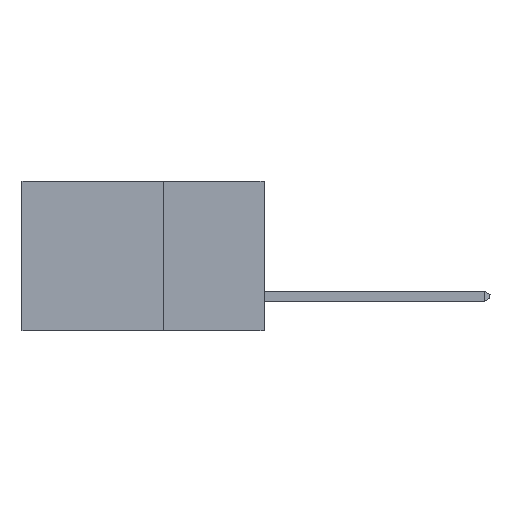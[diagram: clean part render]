
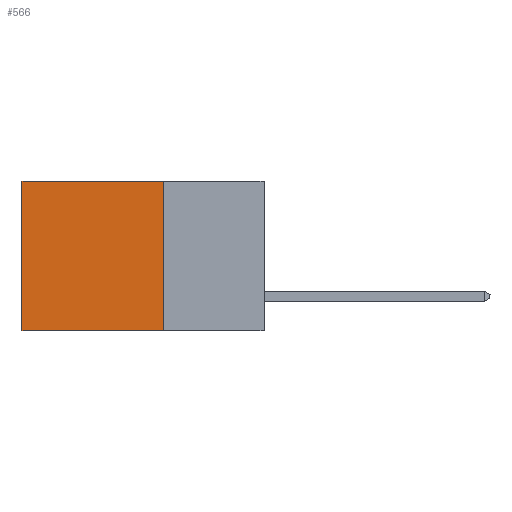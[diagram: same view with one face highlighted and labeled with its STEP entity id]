
A CAD part, left-side view. The second image highlights one B-rep face of the part: STEP entity #566.
In plain terms, the highlighted planar face has unit normal (-1, 0, 0).
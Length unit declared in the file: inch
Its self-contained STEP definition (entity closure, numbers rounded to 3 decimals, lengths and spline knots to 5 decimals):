
#61 = CARTESIAN_POINT ( 'NONE',  ( 0.298, 0.25, -0.37 ) ) ;
#566 = ADVANCED_FACE ( 'NONE', ( #7269 ), #3230, .F. ) ;
#623 = CARTESIAN_POINT ( 'NONE',  ( 0.298, 0.6, 0. ) ) ;
#704 = CARTESIAN_POINT ( 'NONE',  ( 0.298, 0.25, 0. ) ) ;
#1012 = DIRECTION ( 'NONE',  ( 0., 0., -1. ) ) ;
#1106 = LINE ( 'NONE', #704, #5927 ) ;
#1381 = ORIENTED_EDGE ( 'NONE', *, *, #5253, .F. ) ;
#2060 = EDGE_CURVE ( 'NONE', #2412, #5916, #2661, .T. ) ;
#2273 = DIRECTION ( 'NONE',  ( 0., 1., 0. ) ) ;
#2412 = VERTEX_POINT ( 'NONE', #61 ) ;
#2661 = LINE ( 'NONE', #9567, #9022 ) ;
#2744 = VECTOR ( 'NONE', #8785, 39.37008 ) ;
#3144 = VERTEX_POINT ( 'NONE', #4530 ) ;
#3230 = PLANE ( 'NONE',  #8269 ) ;
#3354 = ORIENTED_EDGE ( 'NONE', *, *, #4149, .T. ) ;
#3953 = EDGE_CURVE ( 'NONE', #5698, #5916, #4781, .T. ) ;
#4019 = CARTESIAN_POINT ( 'NONE',  ( 0.298, 0.25, 0. ) ) ;
#4149 = EDGE_CURVE ( 'NONE', #3144, #5698, #1106, .T. ) ;
#4530 = CARTESIAN_POINT ( 'NONE',  ( 0.298, 0.25, 0. ) ) ;
#4781 = LINE ( 'NONE', #7223, #2744 ) ;
#4992 = VECTOR ( 'NONE', #6373, 39.37008 ) ;
#5221 = ORIENTED_EDGE ( 'NONE', *, *, #3953, .T. ) ;
#5253 = EDGE_CURVE ( 'NONE', #3144, #2412, #5700, .T. ) ;
#5552 = DIRECTION ( 'NONE',  ( 1., 0., 0. ) ) ;
#5698 = VERTEX_POINT ( 'NONE', #623 ) ;
#5700 = LINE ( 'NONE', #9438, #4992 ) ;
#5861 = CARTESIAN_POINT ( 'NONE',  ( 0.298, 0.6, -0.37 ) ) ;
#5916 = VERTEX_POINT ( 'NONE', #5861 ) ;
#5927 = VECTOR ( 'NONE', #2273, 39.37008 ) ;
#6181 = EDGE_LOOP ( 'NONE', ( #5221, #9364, #1381, #3354 ) ) ;
#6373 = DIRECTION ( 'NONE',  ( 0., 0., -1. ) ) ;
#7223 = CARTESIAN_POINT ( 'NONE',  ( 0.298, 0.6, 0. ) ) ;
#7269 = FACE_OUTER_BOUND ( 'NONE', #6181, .T. ) ;
#8060 = DIRECTION ( 'NONE',  ( 0., 1., 0. ) ) ;
#8269 = AXIS2_PLACEMENT_3D ( 'NONE', #4019, #5552, #1012 ) ;
#8785 = DIRECTION ( 'NONE',  ( 0., 0., -1. ) ) ;
#9022 = VECTOR ( 'NONE', #8060, 39.37008 ) ;
#9364 = ORIENTED_EDGE ( 'NONE', *, *, #2060, .F. ) ;
#9438 = CARTESIAN_POINT ( 'NONE',  ( 0.298, 0.25, 0. ) ) ;
#9567 = CARTESIAN_POINT ( 'NONE',  ( 0.298, 0.25, -0.37 ) ) ;
